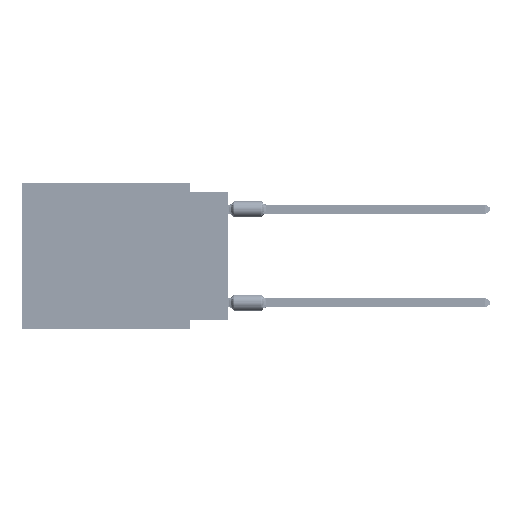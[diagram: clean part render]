
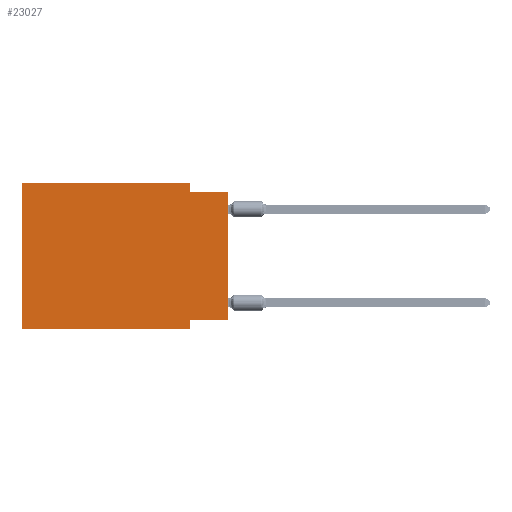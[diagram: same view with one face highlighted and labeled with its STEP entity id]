
A CAD part, left-side view. The second image highlights one B-rep face of the part: STEP entity #23027.
In plain terms, the highlighted planar face has unit normal (-1, 0, 0).
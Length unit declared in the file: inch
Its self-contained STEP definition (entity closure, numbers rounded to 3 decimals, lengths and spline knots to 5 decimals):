
#669 = DIRECTION ( 'NONE',  ( 0., 0., 1. ) ) ;
#918 = ORIENTED_EDGE ( 'NONE', *, *, #67440, .T. ) ;
#943 = CARTESIAN_POINT ( 'NONE',  ( 0., 0.1, 0. ) ) ;
#1155 = CARTESIAN_POINT ( 'NONE',  ( 0., 0., -0.365 ) ) ;
#1178 = ORIENTED_EDGE ( 'NONE', *, *, #77881, .T. ) ;
#2131 = LINE ( 'NONE', #50696, #77938 ) ;
#2812 = ORIENTED_EDGE ( 'NONE', *, *, #83762, .F. ) ;
#2934 = CARTESIAN_POINT ( 'NONE',  ( 0., 0.1, 0. ) ) ;
#3960 = CARTESIAN_POINT ( 'NONE',  ( 0., 0.55, 0. ) ) ;
#5281 = VERTEX_POINT ( 'NONE', #18483 ) ;
#6318 = CARTESIAN_POINT ( 'NONE',  ( 0., 0., -0.365 ) ) ;
#7177 = LINE ( 'NONE', #6318, #7314 ) ;
#7314 = VECTOR ( 'NONE', #33256, 39.37008 ) ;
#7568 = DIRECTION ( 'NONE',  ( 0., 0., -1. ) ) ;
#11174 = VERTEX_POINT ( 'NONE', #13656 ) ;
#13656 = CARTESIAN_POINT ( 'NONE',  ( 0., 0.1, -0.025 ) ) ;
#15522 = LINE ( 'NONE', #943, #75176 ) ;
#18483 = CARTESIAN_POINT ( 'NONE',  ( 0., 0., -0.025 ) ) ;
#21997 = DIRECTION ( 'NONE',  ( 0., 0., -1. ) ) ;
#22800 = LINE ( 'NONE', #55928, #53456 ) ;
#23027 = ADVANCED_FACE ( 'NONE', ( #61410 ), #73360, .F. ) ;
#29923 = CARTESIAN_POINT ( 'NONE',  ( 0., 0.1, -0.39 ) ) ;
#33256 = DIRECTION ( 'NONE',  ( 0., 1., 0. ) ) ;
#34030 = DIRECTION ( 'NONE',  ( 0., 0., -1. ) ) ;
#35394 = EDGE_CURVE ( 'NONE', #53911, #70488, #7177, .T. ) ;
#36737 = EDGE_CURVE ( 'NONE', #72715, #84515, #69539, .T. ) ;
#36860 = ORIENTED_EDGE ( 'NONE', *, *, #36737, .F. ) ;
#37120 = EDGE_CURVE ( 'NONE', #11174, #5281, #81675, .T. ) ;
#37363 = CARTESIAN_POINT ( 'NONE',  ( 0., 0.1, -0.39 ) ) ;
#42164 = EDGE_LOOP ( 'NONE', ( #1178, #71059, #78577, #63078, #36860, #918, #2812, #79748 ) ) ;
#42490 = EDGE_CURVE ( 'NONE', #84515, #48328, #22800, .T. ) ;
#45520 = VERTEX_POINT ( 'NONE', #37363 ) ;
#48143 = CARTESIAN_POINT ( 'NONE',  ( 0., 0., -0.025 ) ) ;
#48328 = VERTEX_POINT ( 'NONE', #2934 ) ;
#49770 = VECTOR ( 'NONE', #669, 39.37008 ) ;
#50696 = CARTESIAN_POINT ( 'NONE',  ( 0., 0.55, -0.39 ) ) ;
#52211 = CARTESIAN_POINT ( 'NONE',  ( 0., 0.1, -0.365 ) ) ;
#53456 = VECTOR ( 'NONE', #56353, 39.37008 ) ;
#53487 = CARTESIAN_POINT ( 'NONE',  ( 0., 0.55, 0. ) ) ;
#53911 = VERTEX_POINT ( 'NONE', #1155 ) ;
#55359 = CARTESIAN_POINT ( 'NONE',  ( 0., 0.55, -0.39 ) ) ;
#55928 = CARTESIAN_POINT ( 'NONE',  ( 0., 0.55, 0. ) ) ;
#56322 = AXIS2_PLACEMENT_3D ( 'NONE', #53487, #60970, #34030 ) ;
#56353 = DIRECTION ( 'NONE',  ( 0., -1., 0. ) ) ;
#60970 = DIRECTION ( 'NONE',  ( 1., 0., 0. ) ) ;
#61410 = FACE_OUTER_BOUND ( 'NONE', #42164, .T. ) ;
#61596 = VECTOR ( 'NONE', #21997, 39.37008 ) ;
#62630 = VECTOR ( 'NONE', #87121, 39.37008 ) ;
#63078 = ORIENTED_EDGE ( 'NONE', *, *, #42490, .F. ) ;
#66825 = CARTESIAN_POINT ( 'NONE',  ( 0., 0., 0. ) ) ;
#67440 = EDGE_CURVE ( 'NONE', #72715, #45520, #2131, .T. ) ;
#69539 = LINE ( 'NONE', #82331, #49770 ) ;
#70488 = VERTEX_POINT ( 'NONE', #52211 ) ;
#71059 = ORIENTED_EDGE ( 'NONE', *, *, #37120, .F. ) ;
#72715 = VERTEX_POINT ( 'NONE', #55359 ) ;
#73360 = PLANE ( 'NONE',  #56322 ) ;
#75072 = DIRECTION ( 'NONE',  ( 0., -1., 0. ) ) ;
#75176 = VECTOR ( 'NONE', #7568, 39.37008 ) ;
#76965 = EDGE_CURVE ( 'NONE', #48328, #11174, #15522, .T. ) ;
#77881 = EDGE_CURVE ( 'NONE', #53911, #5281, #86250, .T. ) ;
#77938 = VECTOR ( 'NONE', #84653, 39.37008 ) ;
#78577 = ORIENTED_EDGE ( 'NONE', *, *, #76965, .F. ) ;
#79431 = VECTOR ( 'NONE', #75072, 39.37008 ) ;
#79748 = ORIENTED_EDGE ( 'NONE', *, *, #35394, .F. ) ;
#81675 = LINE ( 'NONE', #48143, #79431 ) ;
#82331 = CARTESIAN_POINT ( 'NONE',  ( 0., 0.55, 0. ) ) ;
#82460 = LINE ( 'NONE', #29923, #61596 ) ;
#83762 = EDGE_CURVE ( 'NONE', #70488, #45520, #82460, .T. ) ;
#84515 = VERTEX_POINT ( 'NONE', #3960 ) ;
#84653 = DIRECTION ( 'NONE',  ( 0., -1., 0. ) ) ;
#86250 = LINE ( 'NONE', #66825, #62630 ) ;
#87121 = DIRECTION ( 'NONE',  ( 0., 0., 1. ) ) ;
